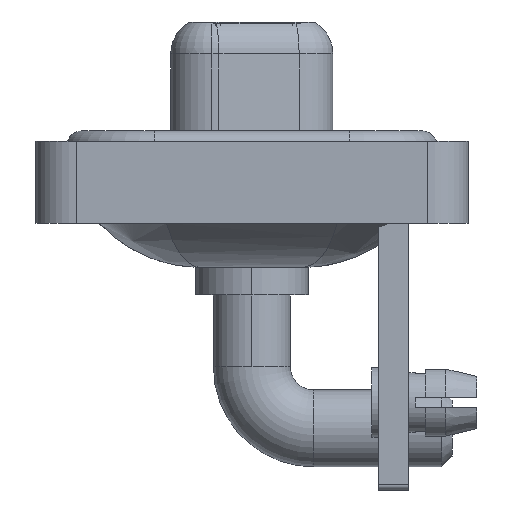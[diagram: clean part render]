
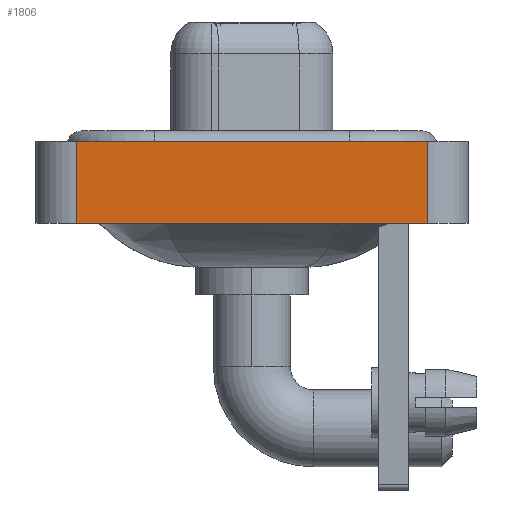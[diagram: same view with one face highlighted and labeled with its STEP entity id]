
A CAD part, left-side view. The second image highlights one B-rep face of the part: STEP entity #1806.
In plain terms, the highlighted planar face has unit normal (-1, 0, 0).
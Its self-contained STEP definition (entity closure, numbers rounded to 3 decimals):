
#635 = VERTEX_POINT ( 'NONE', #2299 ) ;
#942 = LINE ( 'NONE', #12524, #8639 ) ;
#1251 = VERTEX_POINT ( 'NONE', #14045 ) ;
#1806 = ADVANCED_FACE ( 'NONE', ( #4869 ), #3281, .T. ) ;
#1960 = CARTESIAN_POINT ( 'NONE',  ( -7.3, -8.55, -3.6 ) ) ;
#2299 = CARTESIAN_POINT ( 'NONE',  ( -7.3, 8.55, 0.4 ) ) ;
#2435 = LINE ( 'NONE', #18266, #14547 ) ;
#2765 = VERTEX_POINT ( 'NONE', #9005 ) ;
#3153 = EDGE_CURVE ( 'NONE', #15299, #635, #16325, .T. ) ;
#3281 = PLANE ( 'NONE',  #14809 ) ;
#4189 = ORIENTED_EDGE ( 'NONE', *, *, #6568, .T. ) ;
#4869 = FACE_OUTER_BOUND ( 'NONE', #18254, .T. ) ;
#5345 = DIRECTION ( 'NONE',  ( 0., -1., 0. ) ) ;
#5878 = EDGE_CURVE ( 'NONE', #635, #1251, #16287, .T. ) ;
#6240 = DIRECTION ( 'NONE',  ( 0., 0., 1. ) ) ;
#6568 = EDGE_CURVE ( 'NONE', #15299, #2765, #942, .T. ) ;
#6755 = ORIENTED_EDGE ( 'NONE', *, *, #5878, .F. ) ;
#6923 = DIRECTION ( 'NONE',  ( 0., 0., 1. ) ) ;
#7597 = DIRECTION ( 'NONE',  ( 0., -1., 0. ) ) ;
#7731 = CARTESIAN_POINT ( 'NONE',  ( -7.3, 8.55, -3.6 ) ) ;
#8639 = VECTOR ( 'NONE', #5345, 1000. ) ;
#9005 = CARTESIAN_POINT ( 'NONE',  ( -7.3, -8.55, -3.6 ) ) ;
#9197 = ORIENTED_EDGE ( 'NONE', *, *, #11438, .T. ) ;
#9593 = ORIENTED_EDGE ( 'NONE', *, *, #3153, .F. ) ;
#10239 = CARTESIAN_POINT ( 'NONE',  ( -7.3, 8.55, -3.6 ) ) ;
#10478 = DIRECTION ( 'NONE',  ( -1., 0., 0. ) ) ;
#11438 = EDGE_CURVE ( 'NONE', #2765, #1251, #2435, .T. ) ;
#11858 = VECTOR ( 'NONE', #6240, 1000. ) ;
#12524 = CARTESIAN_POINT ( 'NONE',  ( -7.3, -8.55, -3.6 ) ) ;
#12803 = VECTOR ( 'NONE', #7597, 1000. ) ;
#14045 = CARTESIAN_POINT ( 'NONE',  ( -7.3, -8.55, 0.4 ) ) ;
#14547 = VECTOR ( 'NONE', #6923, 1000. ) ;
#14809 = AXIS2_PLACEMENT_3D ( 'NONE', #1960, #10478, #17792 ) ;
#15299 = VERTEX_POINT ( 'NONE', #7731 ) ;
#16287 = LINE ( 'NONE', #17437, #12803 ) ;
#16325 = LINE ( 'NONE', #10239, #11858 ) ;
#17437 = CARTESIAN_POINT ( 'NONE',  ( -7.3, -8.55, 0.4 ) ) ;
#17792 = DIRECTION ( 'NONE',  ( 0., 0., 1. ) ) ;
#18254 = EDGE_LOOP ( 'NONE', ( #9197, #6755, #9593, #4189 ) ) ;
#18266 = CARTESIAN_POINT ( 'NONE',  ( -7.3, -8.55, -3.6 ) ) ;
